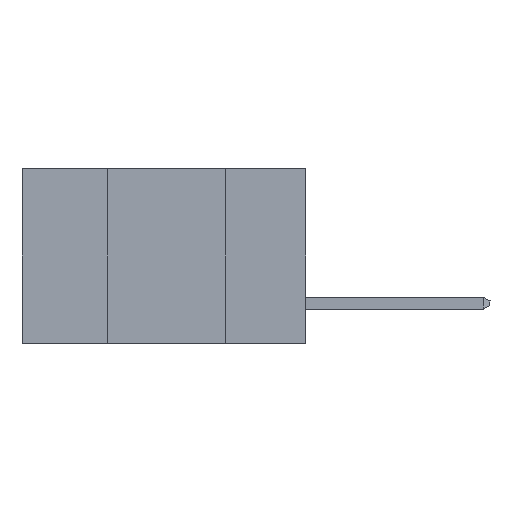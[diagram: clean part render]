
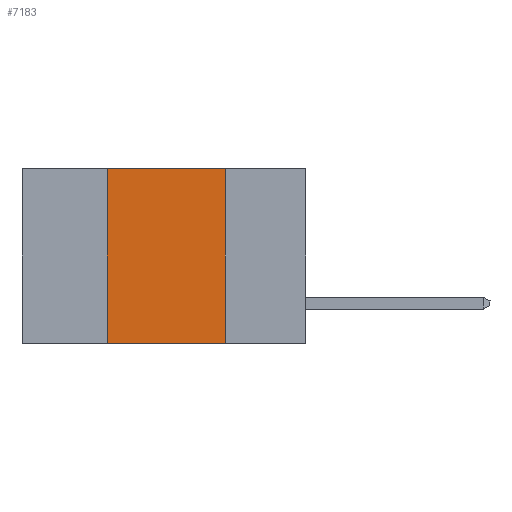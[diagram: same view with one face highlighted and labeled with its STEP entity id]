
A CAD part, left-side view. The second image highlights one B-rep face of the part: STEP entity #7183.
In plain terms, the highlighted planar face has unit normal (-1, 0, 0).
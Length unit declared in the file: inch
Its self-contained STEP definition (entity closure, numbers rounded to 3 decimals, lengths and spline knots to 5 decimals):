
#330 = LINE ( 'NONE', #1522, #5343 ) ;
#809 = CARTESIAN_POINT ( 'NONE',  ( 0., 0.42, -0.37 ) ) ;
#1522 = CARTESIAN_POINT ( 'NONE',  ( 0., 0.6, -0.37 ) ) ;
#5267 = ORIENTED_EDGE ( 'NONE', *, *, #13176, .F. ) ;
#5343 = VECTOR ( 'NONE', #12622, 39.37008 ) ;
#6235 = CARTESIAN_POINT ( 'NONE',  ( 0., 0.42, 0. ) ) ;
#7183 = ADVANCED_FACE ( 'NONE', ( #9473 ), #9219, .F. ) ;
#8143 = ORIENTED_EDGE ( 'NONE', *, *, #24374, .T. ) ;
#8524 = EDGE_CURVE ( 'NONE', #24505, #10892, #14676, .T. ) ;
#9216 = EDGE_LOOP ( 'NONE', ( #23080, #22464, #5267, #8143 ) ) ;
#9219 = PLANE ( 'NONE',  #21306 ) ;
#9305 = DIRECTION ( 'NONE',  ( 0., 0., -1. ) ) ;
#9473 = FACE_OUTER_BOUND ( 'NONE', #9216, .T. ) ;
#10633 = VERTEX_POINT ( 'NONE', #6235 ) ;
#10892 = VERTEX_POINT ( 'NONE', #11489 ) ;
#11489 = CARTESIAN_POINT ( 'NONE',  ( 0., 0.17, -0.37 ) ) ;
#12085 = VERTEX_POINT ( 'NONE', #809 ) ;
#12447 = DIRECTION ( 'NONE',  ( 0., -1., 0. ) ) ;
#12622 = DIRECTION ( 'NONE',  ( 0., -1., 0. ) ) ;
#12963 = VECTOR ( 'NONE', #12447, 39.37008 ) ;
#13176 = EDGE_CURVE ( 'NONE', #12085, #10633, #20169, .T. ) ;
#14676 = LINE ( 'NONE', #23122, #18598 ) ;
#15107 = VECTOR ( 'NONE', #19622, 39.37008 ) ;
#16867 = LINE ( 'NONE', #22406, #12963 ) ;
#18598 = VECTOR ( 'NONE', #20855, 39.37008 ) ;
#18768 = CARTESIAN_POINT ( 'NONE',  ( 0., 0.6, 0. ) ) ;
#19458 = CARTESIAN_POINT ( 'NONE',  ( 0., 0.42, 0. ) ) ;
#19622 = DIRECTION ( 'NONE',  ( 0., 0., 1. ) ) ;
#20169 = LINE ( 'NONE', #19458, #15107 ) ;
#20656 = DIRECTION ( 'NONE',  ( 1., 0., 0. ) ) ;
#20855 = DIRECTION ( 'NONE',  ( 0., 0., -1. ) ) ;
#21306 = AXIS2_PLACEMENT_3D ( 'NONE', #18768, #20656, #9305 ) ;
#22406 = CARTESIAN_POINT ( 'NONE',  ( 0., 0.6, 0. ) ) ;
#22464 = ORIENTED_EDGE ( 'NONE', *, *, #23551, .F. ) ;
#23066 = CARTESIAN_POINT ( 'NONE',  ( 0., 0.17, 0. ) ) ;
#23080 = ORIENTED_EDGE ( 'NONE', *, *, #8524, .F. ) ;
#23122 = CARTESIAN_POINT ( 'NONE',  ( 0., 0.17, 0. ) ) ;
#23551 = EDGE_CURVE ( 'NONE', #10633, #24505, #16867, .T. ) ;
#24374 = EDGE_CURVE ( 'NONE', #12085, #10892, #330, .T. ) ;
#24505 = VERTEX_POINT ( 'NONE', #23066 ) ;
